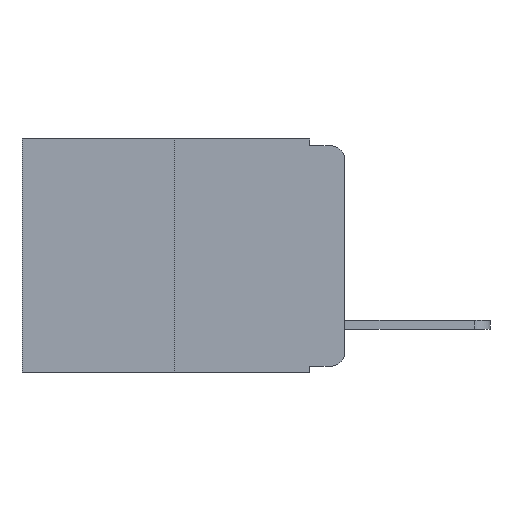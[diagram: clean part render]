
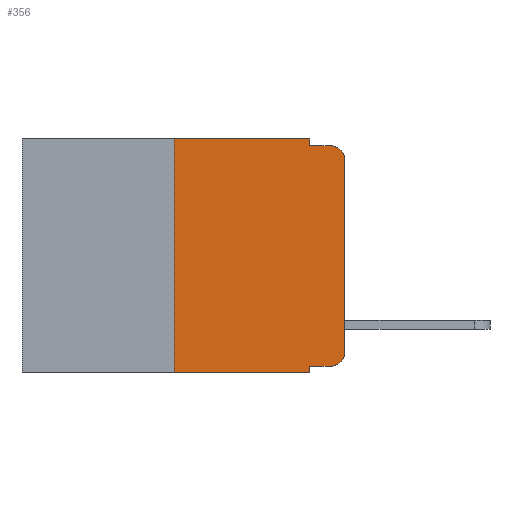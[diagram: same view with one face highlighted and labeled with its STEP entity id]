
A CAD part, left-side view. The second image highlights one B-rep face of the part: STEP entity #356.
In plain terms, the highlighted planar face has unit normal (-1, 0, 0).
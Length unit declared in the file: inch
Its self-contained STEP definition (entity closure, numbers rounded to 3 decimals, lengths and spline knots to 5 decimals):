
#356 = ADVANCED_FACE ( 'NONE', ( #1677 ), #7911, .F. ) ;
#687 = LINE ( 'NONE', #13753, #1347 ) ;
#725 = VERTEX_POINT ( 'NONE', #4646 ) ;
#1328 = DIRECTION ( 'NONE',  ( 0., 0., -1. ) ) ;
#1347 = VECTOR ( 'NONE', #15525, 39.37008 ) ;
#1558 = LINE ( 'NONE', #15191, #11207 ) ;
#1570 = VERTEX_POINT ( 'NONE', #10835 ) ;
#1677 = FACE_OUTER_BOUND ( 'NONE', #20249, .T. ) ;
#1705 = ORIENTED_EDGE ( 'NONE', *, *, #15522, .T. ) ;
#1724 = VERTEX_POINT ( 'NONE', #2379 ) ;
#1816 = CARTESIAN_POINT ( 'NONE',  ( 0., 0.02, -0.333 ) ) ;
#2081 = DIRECTION ( 'NONE',  ( 0., -1., 0. ) ) ;
#2379 = CARTESIAN_POINT ( 'NONE',  ( 0., 0.051, -0.01 ) ) ;
#2749 = ORIENTED_EDGE ( 'NONE', *, *, #12419, .T. ) ;
#2912 = CARTESIAN_POINT ( 'NONE',  ( 0., 0.25, -0.343 ) ) ;
#2917 = DIRECTION ( 'NONE',  ( 0., 0., -1. ) ) ;
#3412 = CARTESIAN_POINT ( 'NONE',  ( 0., 0.473, 0. ) ) ;
#3581 = ORIENTED_EDGE ( 'NONE', *, *, #16009, .F. ) ;
#3786 = CARTESIAN_POINT ( 'NONE',  ( 0., 0.02, -0.03 ) ) ;
#3927 = VERTEX_POINT ( 'NONE', #7687 ) ;
#3981 = VERTEX_POINT ( 'NONE', #15227 ) ;
#4150 = DIRECTION ( 'NONE',  ( 0., -1., 0. ) ) ;
#4646 = CARTESIAN_POINT ( 'NONE',  ( 0., 0., -0.03 ) ) ;
#5149 = CIRCLE ( 'NONE', #10817, 0.02 ) ;
#5746 = DIRECTION ( 'NONE',  ( 0., 0., -1. ) ) ;
#7078 = DIRECTION ( 'NONE',  ( 1., 0., 0. ) ) ;
#7504 = ORIENTED_EDGE ( 'NONE', *, *, #14321, .T. ) ;
#7687 = CARTESIAN_POINT ( 'NONE',  ( 0., 0.051, 0. ) ) ;
#7911 = PLANE ( 'NONE',  #17951 ) ;
#8141 = CARTESIAN_POINT ( 'NONE',  ( 0., 0.02, -0.313 ) ) ;
#9043 = ORIENTED_EDGE ( 'NONE', *, *, #9944, .T. ) ;
#9160 = EDGE_CURVE ( 'NONE', #10094, #17668, #687, .T. ) ;
#9236 = ORIENTED_EDGE ( 'NONE', *, *, #10753, .F. ) ;
#9258 = CARTESIAN_POINT ( 'NONE',  ( 0., 0.051, -0.333 ) ) ;
#9944 = EDGE_CURVE ( 'NONE', #15858, #16560, #22289, .T. ) ;
#10053 = DIRECTION ( 'NONE',  ( 0., 0., -1. ) ) ;
#10094 = VERTEX_POINT ( 'NONE', #2912 ) ;
#10753 = EDGE_CURVE ( 'NONE', #10094, #3981, #19418, .T. ) ;
#10817 = AXIS2_PLACEMENT_3D ( 'NONE', #3786, #16665, #5746 ) ;
#10835 = CARTESIAN_POINT ( 'NONE',  ( 0., 0.02, -0.01 ) ) ;
#10867 = CARTESIAN_POINT ( 'NONE',  ( 0., 0.051, -0.333 ) ) ;
#10882 = LINE ( 'NONE', #12455, #17490 ) ;
#11207 = VECTOR ( 'NONE', #2081, 39.37008 ) ;
#11632 = CARTESIAN_POINT ( 'NONE',  ( 0., 0.473, 0. ) ) ;
#11985 = EDGE_CURVE ( 'NONE', #3927, #1724, #10882, .T. ) ;
#12271 = ORIENTED_EDGE ( 'NONE', *, *, #9160, .T. ) ;
#12419 = EDGE_CURVE ( 'NONE', #21784, #15858, #14221, .T. ) ;
#12455 = CARTESIAN_POINT ( 'NONE',  ( 0., 0.051, 0. ) ) ;
#12456 = ORIENTED_EDGE ( 'NONE', *, *, #13150, .F. ) ;
#12458 = LINE ( 'NONE', #17470, #21603 ) ;
#12982 = DIRECTION ( 'NONE',  ( 0., -1., 0. ) ) ;
#13007 = ORIENTED_EDGE ( 'NONE', *, *, #11985, .F. ) ;
#13150 = EDGE_CURVE ( 'NONE', #1724, #1570, #1558, .T. ) ;
#13677 = VECTOR ( 'NONE', #12982, 39.37008 ) ;
#13753 = CARTESIAN_POINT ( 'NONE',  ( 0., 0.473, -0.343 ) ) ;
#14221 = LINE ( 'NONE', #9258, #13677 ) ;
#14321 = EDGE_CURVE ( 'NONE', #725, #1570, #5149, .T. ) ;
#14457 = VECTOR ( 'NONE', #22903, 39.37008 ) ;
#15191 = CARTESIAN_POINT ( 'NONE',  ( 0., 0.051, -0.01 ) ) ;
#15227 = CARTESIAN_POINT ( 'NONE',  ( 0., 0.25, 0. ) ) ;
#15468 = VECTOR ( 'NONE', #4150, 39.37008 ) ;
#15522 = EDGE_CURVE ( 'NONE', #16560, #725, #12458, .T. ) ;
#15525 = DIRECTION ( 'NONE',  ( 0., -1., 0. ) ) ;
#15858 = VERTEX_POINT ( 'NONE', #1816 ) ;
#16009 = EDGE_CURVE ( 'NONE', #3981, #3927, #20048, .T. ) ;
#16560 = VERTEX_POINT ( 'NONE', #18473 ) ;
#16665 = DIRECTION ( 'NONE',  ( -1., 0., 0. ) ) ;
#16932 = ORIENTED_EDGE ( 'NONE', *, *, #20554, .F. ) ;
#17470 = CARTESIAN_POINT ( 'NONE',  ( 0., 0., 0. ) ) ;
#17490 = VECTOR ( 'NONE', #2917, 39.37008 ) ;
#17668 = VERTEX_POINT ( 'NONE', #22774 ) ;
#17903 = CARTESIAN_POINT ( 'NONE',  ( 0., 0.051, 0. ) ) ;
#17951 = AXIS2_PLACEMENT_3D ( 'NONE', #3412, #7078, #1328 ) ;
#18473 = CARTESIAN_POINT ( 'NONE',  ( 0., 0., -0.313 ) ) ;
#19077 = LINE ( 'NONE', #17903, #14457 ) ;
#19196 = DIRECTION ( 'NONE',  ( 0., 0., 1. ) ) ;
#19418 = LINE ( 'NONE', #19559, #19963 ) ;
#19559 = CARTESIAN_POINT ( 'NONE',  ( 0., 0.25, 0. ) ) ;
#19963 = VECTOR ( 'NONE', #22772, 39.37008 ) ;
#20048 = LINE ( 'NONE', #11632, #15468 ) ;
#20249 = EDGE_LOOP ( 'NONE', ( #1705, #7504, #12456, #13007, #3581, #9236, #12271, #16932, #2749, #9043 ) ) ;
#20554 = EDGE_CURVE ( 'NONE', #21784, #17668, #19077, .T. ) ;
#20572 = DIRECTION ( 'NONE',  ( -1., 0., 0. ) ) ;
#21603 = VECTOR ( 'NONE', #19196, 39.37008 ) ;
#21784 = VERTEX_POINT ( 'NONE', #10867 ) ;
#22289 = CIRCLE ( 'NONE', #22579, 0.02 ) ;
#22579 = AXIS2_PLACEMENT_3D ( 'NONE', #8141, #20572, #10053 ) ;
#22772 = DIRECTION ( 'NONE',  ( 0., 0., 1. ) ) ;
#22774 = CARTESIAN_POINT ( 'NONE',  ( 0., 0.051, -0.343 ) ) ;
#22903 = DIRECTION ( 'NONE',  ( 0., 0., -1. ) ) ;
